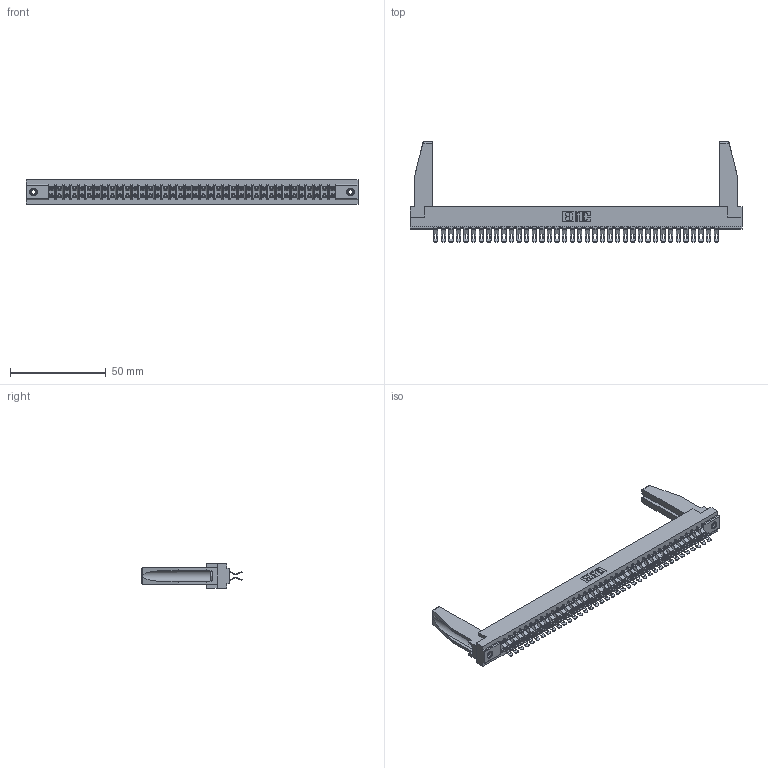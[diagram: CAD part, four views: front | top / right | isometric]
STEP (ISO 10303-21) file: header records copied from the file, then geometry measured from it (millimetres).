
FILE_DESCRIPTION (( 'STEP AP203' ), '1' );
FILE_NAME ('357-076-555-278.STEP', '2019-09-19T13:42:51', ( '' ), ( '' ), 'SwSTEP 2.0', 'SolidWorks 2016', '' );
FILE_SCHEMA (( 'CONFIG_CONTROL_DESIGN' ));
Length unit declared in the file: inch
Products named in the file (5): 307-290-001_555; 345-250-001_345-250-001-102; 357-076-555-278; 307 Part_.156 Dia Mounting Holes; 307-220-078
Assembly tree (81 placements, depth 2):
  357-076-555-278
    307 Part_.156 Dia Mounting Holes
    307-290-001_555  x76
    307-220-078  x2
    345-250-001_345-250-001-102  x2
Bounding box: 173.58 x 52.45 x 12.7 mm (x, y, z)
Volume: 22650 mm3; surface area: 27830.1 mm2
Topology: 81 solids, 81 shells, 4923 faces, 14409 edges, 9390 vertices
Faces by surface type: plane 2738, cylinder 2091, sphere 78, cone 12, torus 4
Entity records: 37262 total; most frequent: CARTESIAN_POINT 6112, ORIENTED_EDGE 6018, DIRECTION 5949, EDGE_CURVE 3009, VECTOR 2299, LINE 2299, VERTEX_POINT 1946, AXIS2_PLACEMENT_3D 1825
